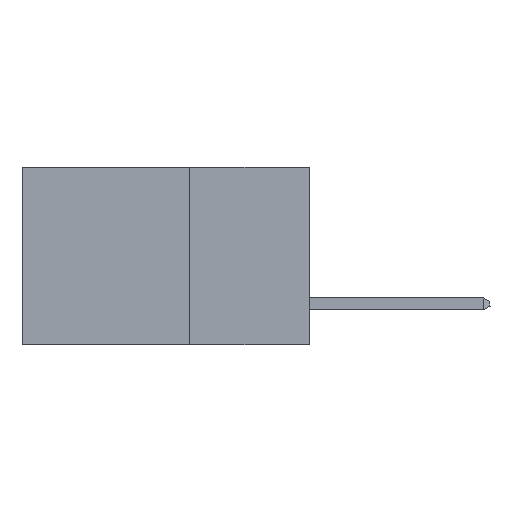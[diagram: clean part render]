
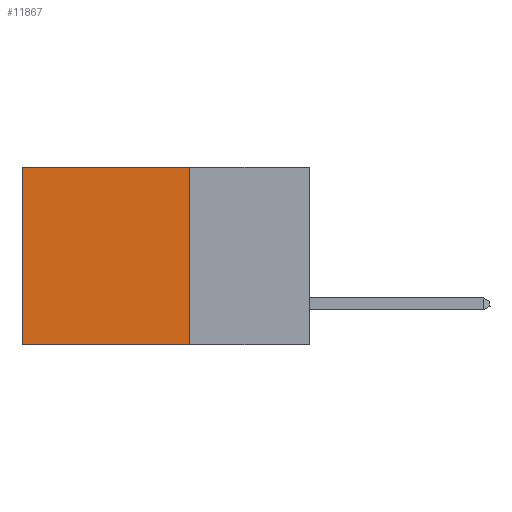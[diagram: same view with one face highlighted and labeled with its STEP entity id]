
A CAD part, left-side view. The second image highlights one B-rep face of the part: STEP entity #11867.
In plain terms, the highlighted planar face has unit normal (-1, 0, 0).
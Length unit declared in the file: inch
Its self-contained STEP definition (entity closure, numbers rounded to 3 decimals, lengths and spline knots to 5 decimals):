
#1634 = CARTESIAN_POINT ( 'NONE',  ( 0.2875, 0.25, 0. ) ) ;
#2093 = LINE ( 'NONE', #32336, #9783 ) ;
#4924 = DIRECTION ( 'NONE',  ( 0., 0., -1. ) ) ;
#5790 = VECTOR ( 'NONE', #4924, 39.37008 ) ;
#6568 = CARTESIAN_POINT ( 'NONE',  ( 0.2875, 0.6, -0.37 ) ) ;
#7202 = EDGE_CURVE ( 'NONE', #13954, #30955, #24530, .T. ) ;
#9197 = EDGE_CURVE ( 'NONE', #29783, #45549, #30827, .T. ) ;
#9783 = VECTOR ( 'NONE', #30650, 39.37008 ) ;
#11365 = CARTESIAN_POINT ( 'NONE',  ( 0.2875, 0.25, 0. ) ) ;
#11609 = ORIENTED_EDGE ( 'NONE', *, *, #9197, .F. ) ;
#11867 = ADVANCED_FACE ( 'NONE', ( #29243 ), #43501, .F. ) ;
#13954 = VERTEX_POINT ( 'NONE', #28034 ) ;
#19129 = EDGE_LOOP ( 'NONE', ( #38065, #11609, #42022, #43131 ) ) ;
#20739 = VECTOR ( 'NONE', #33446, 39.37008 ) ;
#21254 = LINE ( 'NONE', #1634, #5790 ) ;
#23330 = VECTOR ( 'NONE', #25924, 39.37008 ) ;
#24530 = LINE ( 'NONE', #11365, #23330 ) ;
#25300 = AXIS2_PLACEMENT_3D ( 'NONE', #36088, #28359, #47771 ) ;
#25924 = DIRECTION ( 'NONE',  ( 0., 1., 0. ) ) ;
#28034 = CARTESIAN_POINT ( 'NONE',  ( 0.2875, 0.25, 0. ) ) ;
#28359 = DIRECTION ( 'NONE',  ( 1., 0., 0. ) ) ;
#29243 = FACE_OUTER_BOUND ( 'NONE', #19129, .T. ) ;
#29654 = CARTESIAN_POINT ( 'NONE',  ( 0.2875, 0.25, -0.37 ) ) ;
#29783 = VERTEX_POINT ( 'NONE', #48614 ) ;
#30650 = DIRECTION ( 'NONE',  ( 0., 0., -1. ) ) ;
#30827 = LINE ( 'NONE', #29654, #20739 ) ;
#30955 = VERTEX_POINT ( 'NONE', #35569 ) ;
#31509 = EDGE_CURVE ( 'NONE', #30955, #45549, #2093, .T. ) ;
#32336 = CARTESIAN_POINT ( 'NONE',  ( 0.2875, 0.6, 0. ) ) ;
#33446 = DIRECTION ( 'NONE',  ( 0., 1., 0. ) ) ;
#35569 = CARTESIAN_POINT ( 'NONE',  ( 0.2875, 0.6, 0. ) ) ;
#36088 = CARTESIAN_POINT ( 'NONE',  ( 0.2875, 0.25, 0. ) ) ;
#38065 = ORIENTED_EDGE ( 'NONE', *, *, #31509, .T. ) ;
#42022 = ORIENTED_EDGE ( 'NONE', *, *, #45312, .F. ) ;
#43131 = ORIENTED_EDGE ( 'NONE', *, *, #7202, .T. ) ;
#43501 = PLANE ( 'NONE',  #25300 ) ;
#45312 = EDGE_CURVE ( 'NONE', #13954, #29783, #21254, .T. ) ;
#45549 = VERTEX_POINT ( 'NONE', #6568 ) ;
#47771 = DIRECTION ( 'NONE',  ( 0., 0., -1. ) ) ;
#48614 = CARTESIAN_POINT ( 'NONE',  ( 0.2875, 0.25, -0.37 ) ) ;
